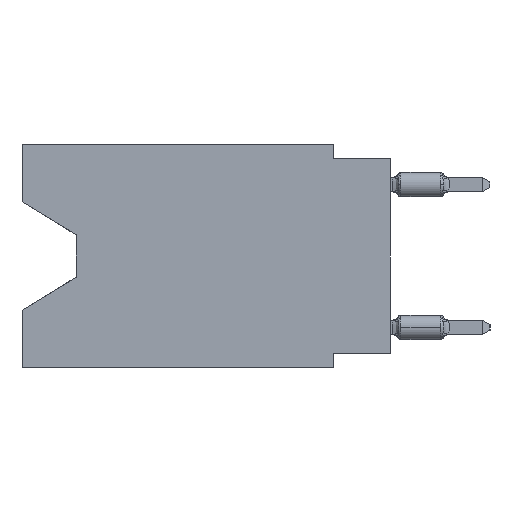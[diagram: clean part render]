
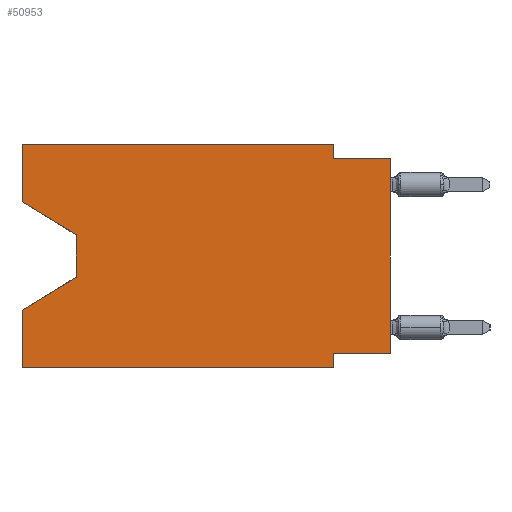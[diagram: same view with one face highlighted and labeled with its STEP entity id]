
A CAD part, left-side view. The second image highlights one B-rep face of the part: STEP entity #50953.
In plain terms, the highlighted planar face has unit normal (-1, 0, 0).
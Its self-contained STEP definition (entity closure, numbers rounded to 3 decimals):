
#2147 = EDGE_CURVE ( 'NONE', #51997, #14714, #36047, .T. ) ;
#2960 = CARTESIAN_POINT ( 'NONE',  ( 0., 16.383, 0. ) ) ;
#3321 = EDGE_CURVE ( 'NONE', #45946, #57673, #32114, .T. ) ;
#3615 = ORIENTED_EDGE ( 'NONE', *, *, #9713, .T. ) ;
#4235 = ORIENTED_EDGE ( 'NONE', *, *, #4276, .F. ) ;
#4276 = EDGE_CURVE ( 'NONE', #57673, #24984, #12867, .T. ) ;
#5981 = LINE ( 'NONE', #16422, #53486 ) ;
#6194 = EDGE_CURVE ( 'NONE', #31941, #33496, #35745, .T. ) ;
#6387 = VERTEX_POINT ( 'NONE', #51059 ) ;
#7146 = CARTESIAN_POINT ( 'NONE',  ( 0., 2.54, -9.906 ) ) ;
#8031 = DIRECTION ( 'NONE',  ( 0., 0.855, -0.519 ) ) ;
#8063 = DIRECTION ( 'NONE',  ( 0., 0., -1. ) ) ;
#8182 = CARTESIAN_POINT ( 'NONE',  ( 0., 16.383, -9.906 ) ) ;
#8487 = DIRECTION ( 'NONE',  ( 0., -1., 0. ) ) ;
#8491 = DIRECTION ( 'NONE',  ( 0., 0., 1. ) ) ;
#9569 = DIRECTION ( 'NONE',  ( 1., 0., 0. ) ) ;
#9713 = EDGE_CURVE ( 'NONE', #59791, #14714, #52601, .T. ) ;
#10123 = ORIENTED_EDGE ( 'NONE', *, *, #31029, .F. ) ;
#10409 = VECTOR ( 'NONE', #50451, 1000. ) ;
#12652 = DIRECTION ( 'NONE',  ( 0., 0., -1. ) ) ;
#12867 = LINE ( 'NONE', #31284, #29223 ) ;
#12981 = CARTESIAN_POINT ( 'NONE',  ( 0., 16.383, -2.546 ) ) ;
#13279 = ORIENTED_EDGE ( 'NONE', *, *, #30416, .T. ) ;
#14714 = VERTEX_POINT ( 'NONE', #41206 ) ;
#15000 = CARTESIAN_POINT ( 'NONE',  ( 0., 2.54, 0. ) ) ;
#16422 = CARTESIAN_POINT ( 'NONE',  ( 0., 16.383, -2.546 ) ) ;
#16776 = LINE ( 'NONE', #25974, #35804 ) ;
#17903 = LINE ( 'NONE', #28322, #44410 ) ;
#19955 = CARTESIAN_POINT ( 'NONE',  ( 0., 2.54, 0. ) ) ;
#21326 = VECTOR ( 'NONE', #12652, 1000. ) ;
#22064 = VECTOR ( 'NONE', #8487, 1000. ) ;
#23200 = ORIENTED_EDGE ( 'NONE', *, *, #44516, .F. ) ;
#23424 = VERTEX_POINT ( 'NONE', #37086 ) ;
#24696 = CARTESIAN_POINT ( 'NONE',  ( 0., 13.97, -5.893 ) ) ;
#24984 = VERTEX_POINT ( 'NONE', #19955 ) ;
#25749 = VECTOR ( 'NONE', #8031, 1000. ) ;
#25974 = CARTESIAN_POINT ( 'NONE',  ( 0., 0., -0.635 ) ) ;
#26098 = CARTESIAN_POINT ( 'NONE',  ( 0., 16.383, 0. ) ) ;
#26763 = CARTESIAN_POINT ( 'NONE',  ( 0., 13.97, -4.013 ) ) ;
#26788 = EDGE_CURVE ( 'NONE', #31941, #23424, #17903, .T. ) ;
#27109 = DIRECTION ( 'NONE',  ( 0., 0., 1. ) ) ;
#27158 = DIRECTION ( 'NONE',  ( 0., 1., 0. ) ) ;
#27288 = CARTESIAN_POINT ( 'NONE',  ( 0., 2.54, -0.635 ) ) ;
#28322 = CARTESIAN_POINT ( 'NONE',  ( 0., 0., 0. ) ) ;
#28832 = VECTOR ( 'NONE', #33704, 1000. ) ;
#29223 = VECTOR ( 'NONE', #50587, 1000. ) ;
#29553 = AXIS2_PLACEMENT_3D ( 'NONE', #46048, #9569, #40834 ) ;
#29883 = ORIENTED_EDGE ( 'NONE', *, *, #3321, .F. ) ;
#30416 = EDGE_CURVE ( 'NONE', #51997, #32091, #50183, .T. ) ;
#30467 = EDGE_LOOP ( 'NONE', ( #45480, #47935, #3615, #58815, #13279, #23200, #37720, #39487, #10123, #58896, #4235, #29883 ) ) ;
#30772 = LINE ( 'NONE', #7146, #37797 ) ;
#31029 = EDGE_CURVE ( 'NONE', #33718, #23424, #16776, .T. ) ;
#31284 = CARTESIAN_POINT ( 'NONE',  ( 0., 16.383, 0. ) ) ;
#31941 = VERTEX_POINT ( 'NONE', #41351 ) ;
#32091 = VERTEX_POINT ( 'NONE', #57566 ) ;
#32114 = LINE ( 'NONE', #2960, #36998 ) ;
#33496 = VERTEX_POINT ( 'NONE', #59154 ) ;
#33704 = DIRECTION ( 'NONE',  ( 0., 0., -1. ) ) ;
#33718 = VERTEX_POINT ( 'NONE', #27288 ) ;
#35745 = LINE ( 'NONE', #50134, #47081 ) ;
#35804 = VECTOR ( 'NONE', #58755, 1000. ) ;
#36047 = LINE ( 'NONE', #55952, #10409 ) ;
#36998 = VECTOR ( 'NONE', #8491, 1000. ) ;
#37086 = CARTESIAN_POINT ( 'NONE',  ( 0., 0., -0.635 ) ) ;
#37720 = ORIENTED_EDGE ( 'NONE', *, *, #6194, .F. ) ;
#37797 = VECTOR ( 'NONE', #8063, 1000. ) ;
#37930 = CARTESIAN_POINT ( 'NONE',  ( 0., 13.97, -5.893 ) ) ;
#38760 = EDGE_CURVE ( 'NONE', #24984, #33718, #56985, .T. ) ;
#39487 = ORIENTED_EDGE ( 'NONE', *, *, #26788, .T. ) ;
#40834 = DIRECTION ( 'NONE',  ( 0., 0., -1. ) ) ;
#41206 = CARTESIAN_POINT ( 'NONE',  ( 0., 16.383, -7.36 ) ) ;
#41351 = CARTESIAN_POINT ( 'NONE',  ( 0., 0., -9.271 ) ) ;
#44303 = DIRECTION ( 'NONE',  ( 0., -0.855, -0.519 ) ) ;
#44410 = VECTOR ( 'NONE', #27109, 1000. ) ;
#44516 = EDGE_CURVE ( 'NONE', #33496, #32091, #30772, .T. ) ;
#45480 = ORIENTED_EDGE ( 'NONE', *, *, #58672, .T. ) ;
#45946 = VERTEX_POINT ( 'NONE', #12981 ) ;
#46048 = CARTESIAN_POINT ( 'NONE',  ( 0., 16.383, 0. ) ) ;
#47081 = VECTOR ( 'NONE', #27158, 1000. ) ;
#47935 = ORIENTED_EDGE ( 'NONE', *, *, #60428, .T. ) ;
#50134 = CARTESIAN_POINT ( 'NONE',  ( 0., 0., -9.271 ) ) ;
#50183 = LINE ( 'NONE', #8182, #22064 ) ;
#50451 = DIRECTION ( 'NONE',  ( 0., 0., 1. ) ) ;
#50587 = DIRECTION ( 'NONE',  ( 0., -1., 0. ) ) ;
#50953 = ADVANCED_FACE ( 'NONE', ( #56157 ), #50965, .F. ) ;
#50965 = PLANE ( 'NONE',  #29553 ) ;
#51059 = CARTESIAN_POINT ( 'NONE',  ( 0., 13.97, -4.013 ) ) ;
#51997 = VERTEX_POINT ( 'NONE', #53814 ) ;
#52601 = LINE ( 'NONE', #24696, #25749 ) ;
#53486 = VECTOR ( 'NONE', #44303, 1000. ) ;
#53814 = CARTESIAN_POINT ( 'NONE',  ( 0., 16.383, -9.906 ) ) ;
#54961 = LINE ( 'NONE', #26763, #21326 ) ;
#55952 = CARTESIAN_POINT ( 'NONE',  ( 0., 16.383, 0. ) ) ;
#56157 = FACE_OUTER_BOUND ( 'NONE', #30467, .T. ) ;
#56985 = LINE ( 'NONE', #15000, #28832 ) ;
#57566 = CARTESIAN_POINT ( 'NONE',  ( 0., 2.54, -9.906 ) ) ;
#57673 = VERTEX_POINT ( 'NONE', #26098 ) ;
#58672 = EDGE_CURVE ( 'NONE', #45946, #6387, #5981, .T. ) ;
#58755 = DIRECTION ( 'NONE',  ( 0., -1., 0. ) ) ;
#58815 = ORIENTED_EDGE ( 'NONE', *, *, #2147, .F. ) ;
#58896 = ORIENTED_EDGE ( 'NONE', *, *, #38760, .F. ) ;
#59154 = CARTESIAN_POINT ( 'NONE',  ( 0., 2.54, -9.271 ) ) ;
#59791 = VERTEX_POINT ( 'NONE', #37930 ) ;
#60428 = EDGE_CURVE ( 'NONE', #6387, #59791, #54961, .T. ) ;
